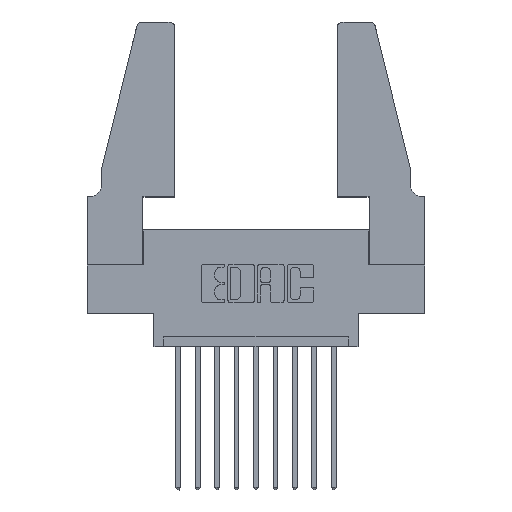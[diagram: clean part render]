
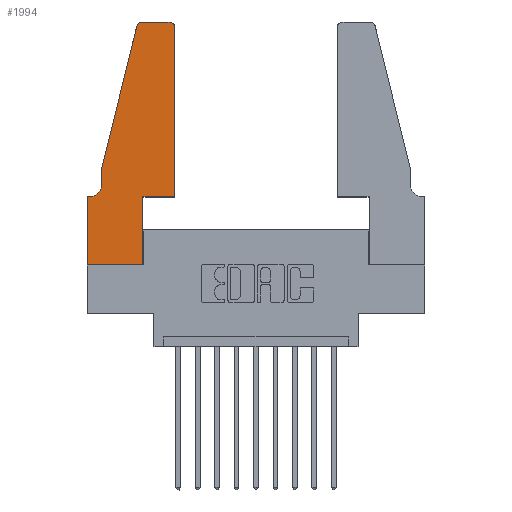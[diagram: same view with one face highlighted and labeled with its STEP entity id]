
A CAD part, top view. The second image highlights one B-rep face of the part: STEP entity #1994.
In plain terms, the highlighted planar face has unit normal (0, 0, 1).
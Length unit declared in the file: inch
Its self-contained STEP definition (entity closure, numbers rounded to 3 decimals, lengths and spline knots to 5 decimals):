
#192 = VERTEX_POINT ( 'NONE', #8441 ) ;
#252 = CARTESIAN_POINT ( 'NONE',  ( 0.0755, 0.5, 0.37 ) ) ;
#410 = AXIS2_PLACEMENT_3D ( 'NONE', #11892, #7832, #3683 ) ;
#467 = EDGE_CURVE ( 'NONE', #10693, #745, #8527, .T. ) ;
#745 = VERTEX_POINT ( 'NONE', #1240 ) ;
#945 = VERTEX_POINT ( 'NONE', #1825 ) ;
#1085 = VECTOR ( 'NONE', #13407, 39.37008 ) ;
#1240 = CARTESIAN_POINT ( 'NONE',  ( 0., 0., 0.37 ) ) ;
#1332 = ORIENTED_EDGE ( 'NONE', *, *, #11133, .T. ) ;
#1486 = CARTESIAN_POINT ( 'NONE',  ( 0.284, 1.22, 0.37 ) ) ;
#1669 = LINE ( 'NONE', #3167, #2636 ) ;
#1780 = CARTESIAN_POINT ( 'NONE',  ( 0.4505, 0.35, 0.37 ) ) ;
#1809 = LINE ( 'NONE', #12037, #12583 ) ;
#1825 = CARTESIAN_POINT ( 'NONE',  ( 0.0055, 0.35, 0.37 ) ) ;
#1994 = ADVANCED_FACE ( 'NONE', ( #11567 ), #10835, .T. ) ;
#2054 = VERTEX_POINT ( 'NONE', #3638 ) ;
#2154 = DIRECTION ( 'NONE',  ( 0., 0., -1. ) ) ;
#2170 = VERTEX_POINT ( 'NONE', #11116 ) ;
#2409 = DIRECTION ( 'NONE',  ( 0., -1., 0. ) ) ;
#2435 = DIRECTION ( 'NONE',  ( 0., 0., 1. ) ) ;
#2500 = AXIS2_PLACEMENT_3D ( 'NONE', #2771, #8123, #4906 ) ;
#2636 = VECTOR ( 'NONE', #9246, 39.37008 ) ;
#2771 = CARTESIAN_POINT ( 'NONE',  ( 0.4205, 1.22, 0.37 ) ) ;
#2798 = EDGE_CURVE ( 'NONE', #12029, #9509, #6667, .T. ) ;
#2860 = CARTESIAN_POINT ( 'NONE',  ( 0.284, 1.25, 0.37 ) ) ;
#2909 = CARTESIAN_POINT ( 'NONE',  ( 0.2865, 0.35, 0.37 ) ) ;
#2975 = ORIENTED_EDGE ( 'NONE', *, *, #9711, .T. ) ;
#3060 = DIRECTION ( 'NONE',  ( -1., 0., 0. ) ) ;
#3167 = CARTESIAN_POINT ( 'NONE',  ( 0.4505, 0.35, 0.37 ) ) ;
#3397 = EDGE_CURVE ( 'NONE', #9509, #6511, #8438, .T. ) ;
#3411 = ORIENTED_EDGE ( 'NONE', *, *, #5236, .T. ) ;
#3501 = EDGE_CURVE ( 'NONE', #2054, #8534, #11216, .T. ) ;
#3638 = CARTESIAN_POINT ( 'NONE',  ( 0.4205, 1.25, 0.37 ) ) ;
#3642 = CARTESIAN_POINT ( 'NONE',  ( 0.0755, 0.42, 0.37 ) ) ;
#3683 = DIRECTION ( 'NONE',  ( 1., 0., 0. ) ) ;
#3706 = CIRCLE ( 'NONE', #12388, 0.03 ) ;
#3976 = VECTOR ( 'NONE', #11332, 39.37008 ) ;
#4030 = ORIENTED_EDGE ( 'NONE', *, *, #4849, .T. ) ;
#4077 = DIRECTION ( 'NONE',  ( -0.239, -0.971, 0. ) ) ;
#4137 = ORIENTED_EDGE ( 'NONE', *, *, #7538, .T. ) ;
#4303 = DIRECTION ( 'NONE',  ( -1., 0., 0. ) ) ;
#4338 = CIRCLE ( 'NONE', #2500, 0.03 ) ;
#4376 = CARTESIAN_POINT ( 'NONE',  ( 0.0055, 0.42, 0.37 ) ) ;
#4849 = EDGE_CURVE ( 'NONE', #7129, #945, #5133, .T. ) ;
#4906 = DIRECTION ( 'NONE',  ( 1., 0., 0. ) ) ;
#5133 = CIRCLE ( 'NONE', #5707, 0.07 ) ;
#5167 = ORIENTED_EDGE ( 'NONE', *, *, #3397, .T. ) ;
#5236 = EDGE_CURVE ( 'NONE', #745, #12029, #6769, .T. ) ;
#5340 = VECTOR ( 'NONE', #13544, 39.37008 ) ;
#5537 = EDGE_CURVE ( 'NONE', #6511, #12106, #1669, .T. ) ;
#5676 = VECTOR ( 'NONE', #4303, 39.37008 ) ;
#5707 = AXIS2_PLACEMENT_3D ( 'NONE', #4376, #2154, #7429 ) ;
#6099 = EDGE_CURVE ( 'NONE', #192, #7129, #1809, .T. ) ;
#6511 = VERTEX_POINT ( 'NONE', #7158 ) ;
#6667 = LINE ( 'NONE', #2909, #1085 ) ;
#6769 = LINE ( 'NONE', #9181, #3976 ) ;
#7129 = VERTEX_POINT ( 'NONE', #3642 ) ;
#7158 = CARTESIAN_POINT ( 'NONE',  ( 0.4505, 0.35, 0.37 ) ) ;
#7429 = DIRECTION ( 'NONE',  ( -1., 0., 0. ) ) ;
#7538 = EDGE_CURVE ( 'NONE', #945, #10693, #8826, .T. ) ;
#7829 = ORIENTED_EDGE ( 'NONE', *, *, #5537, .T. ) ;
#7832 = DIRECTION ( 'NONE',  ( 0., 0., 1. ) ) ;
#8103 = VECTOR ( 'NONE', #4077, 39.37008 ) ;
#8123 = DIRECTION ( 'NONE',  ( 0., 0., 1. ) ) ;
#8160 = DIRECTION ( 'NONE',  ( 0., -1., 0. ) ) ;
#8438 = LINE ( 'NONE', #1780, #5340 ) ;
#8441 = CARTESIAN_POINT ( 'NONE',  ( 0.0755, 0.5, 0.37 ) ) ;
#8455 = ORIENTED_EDGE ( 'NONE', *, *, #3501, .T. ) ;
#8527 = LINE ( 'NONE', #12356, #11618 ) ;
#8534 = VERTEX_POINT ( 'NONE', #2860 ) ;
#8537 = CARTESIAN_POINT ( 'NONE',  ( 0.2865, 0., 0.37 ) ) ;
#8707 = DIRECTION ( 'NONE',  ( 1., 0., 0. ) ) ;
#8716 = ORIENTED_EDGE ( 'NONE', *, *, #6099, .T. ) ;
#8826 = LINE ( 'NONE', #9315, #10592 ) ;
#9033 = ORIENTED_EDGE ( 'NONE', *, *, #11442, .T. ) ;
#9181 = CARTESIAN_POINT ( 'NONE',  ( 0., 0., 0.37 ) ) ;
#9246 = DIRECTION ( 'NONE',  ( 0., 1., 0. ) ) ;
#9315 = CARTESIAN_POINT ( 'NONE',  ( 0.0755, 0.35, 0.37 ) ) ;
#9509 = VERTEX_POINT ( 'NONE', #10937 ) ;
#9668 = ORIENTED_EDGE ( 'NONE', *, *, #467, .T. ) ;
#9711 = EDGE_CURVE ( 'NONE', #2170, #192, #11033, .T. ) ;
#9865 = CARTESIAN_POINT ( 'NONE',  ( 0., 0.35, 0.37 ) ) ;
#10537 = CARTESIAN_POINT ( 'NONE',  ( 0.2605, 1.25, 0.37 ) ) ;
#10592 = VECTOR ( 'NONE', #3060, 39.37008 ) ;
#10693 = VERTEX_POINT ( 'NONE', #9865 ) ;
#10835 = PLANE ( 'NONE',  #410 ) ;
#10937 = CARTESIAN_POINT ( 'NONE',  ( 0.2865, 0.35, 0.37 ) ) ;
#11033 = LINE ( 'NONE', #252, #8103 ) ;
#11116 = CARTESIAN_POINT ( 'NONE',  ( 0.25487, 1.22718, 0.37 ) ) ;
#11133 = EDGE_CURVE ( 'NONE', #8534, #2170, #3706, .T. ) ;
#11216 = LINE ( 'NONE', #10537, #5676 ) ;
#11332 = DIRECTION ( 'NONE',  ( 1., 0., 0. ) ) ;
#11442 = EDGE_CURVE ( 'NONE', #12106, #2054, #4338, .T. ) ;
#11567 = FACE_OUTER_BOUND ( 'NONE', #13075, .T. ) ;
#11618 = VECTOR ( 'NONE', #8160, 39.37008 ) ;
#11634 = CARTESIAN_POINT ( 'NONE',  ( 0.4505, 1.22, 0.37 ) ) ;
#11892 = CARTESIAN_POINT ( 'NONE',  ( 0., 0.35, 0.37 ) ) ;
#12029 = VERTEX_POINT ( 'NONE', #8537 ) ;
#12037 = CARTESIAN_POINT ( 'NONE',  ( 0.0755, 0.5, 0.37 ) ) ;
#12106 = VERTEX_POINT ( 'NONE', #11634 ) ;
#12356 = CARTESIAN_POINT ( 'NONE',  ( 0., 0., 0.37 ) ) ;
#12388 = AXIS2_PLACEMENT_3D ( 'NONE', #1486, #2435, #8707 ) ;
#12471 = ORIENTED_EDGE ( 'NONE', *, *, #2798, .T. ) ;
#12583 = VECTOR ( 'NONE', #2409, 39.37008 ) ;
#13075 = EDGE_LOOP ( 'NONE', ( #8455, #1332, #2975, #8716, #4030, #4137, #9668, #3411, #12471, #5167, #7829, #9033 ) ) ;
#13407 = DIRECTION ( 'NONE',  ( 0., 1., 0. ) ) ;
#13544 = DIRECTION ( 'NONE',  ( 1., 0., 0. ) ) ;
